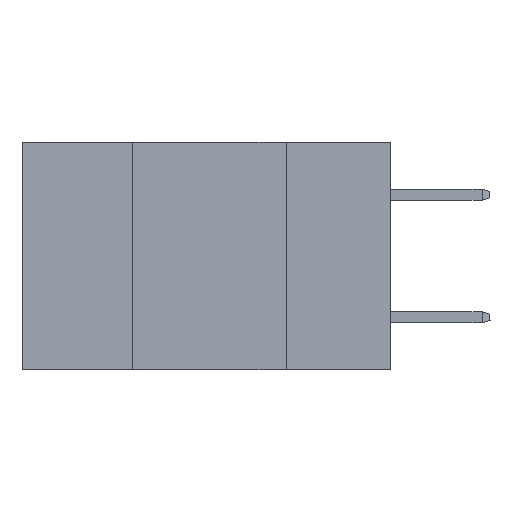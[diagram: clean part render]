
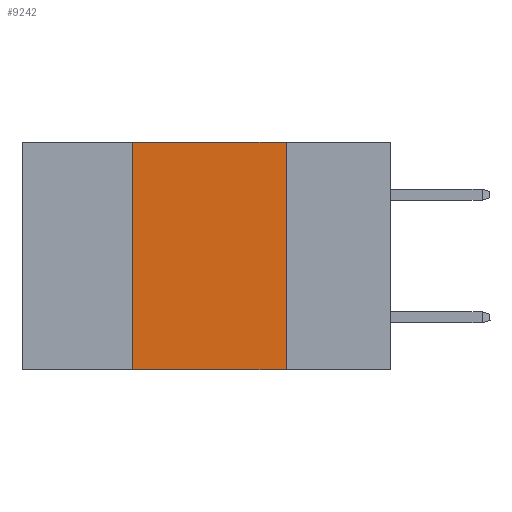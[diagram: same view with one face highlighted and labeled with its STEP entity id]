
A CAD part, left-side view. The second image highlights one B-rep face of the part: STEP entity #9242.
In plain terms, the highlighted planar face has unit normal (-1, 0, 0).
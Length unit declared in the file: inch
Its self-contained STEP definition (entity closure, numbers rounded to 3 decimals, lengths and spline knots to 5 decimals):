
#1092 = EDGE_CURVE ( 'NONE', #11056, #17982, #3952, .T. ) ;
#1175 = DIRECTION ( 'NONE',  ( 1., 0., 0. ) ) ;
#1371 = DIRECTION ( 'NONE',  ( 0., 0., -1. ) ) ;
#1800 = CARTESIAN_POINT ( 'NONE',  ( 0., 0.42, -0.37 ) ) ;
#2839 = VECTOR ( 'NONE', #8505, 39.37008 ) ;
#3799 = ORIENTED_EDGE ( 'NONE', *, *, #16198, .F. ) ;
#3952 = LINE ( 'NONE', #16289, #2839 ) ;
#5340 = EDGE_LOOP ( 'NONE', ( #8524, #3799, #18509, #17405 ) ) ;
#5628 = LINE ( 'NONE', #19074, #18028 ) ;
#5775 = CARTESIAN_POINT ( 'NONE',  ( 0., 0.17, 0. ) ) ;
#7047 = DIRECTION ( 'NONE',  ( 0., 0., 1. ) ) ;
#7302 = FACE_OUTER_BOUND ( 'NONE', #5340, .T. ) ;
#7561 = AXIS2_PLACEMENT_3D ( 'NONE', #8721, #1175, #1371 ) ;
#8074 = CARTESIAN_POINT ( 'NONE',  ( 0., 0.6, 0. ) ) ;
#8477 = VERTEX_POINT ( 'NONE', #1800 ) ;
#8505 = DIRECTION ( 'NONE',  ( 0., 0., -1. ) ) ;
#8524 = ORIENTED_EDGE ( 'NONE', *, *, #1092, .F. ) ;
#8721 = CARTESIAN_POINT ( 'NONE',  ( 0., 0.6, 0. ) ) ;
#9242 = ADVANCED_FACE ( 'NONE', ( #7302 ), #13471, .F. ) ;
#11056 = VERTEX_POINT ( 'NONE', #5775 ) ;
#11897 = LINE ( 'NONE', #18059, #19009 ) ;
#12640 = DIRECTION ( 'NONE',  ( 0., -1., 0. ) ) ;
#13471 = PLANE ( 'NONE',  #7561 ) ;
#13657 = VERTEX_POINT ( 'NONE', #16832 ) ;
#13703 = DIRECTION ( 'NONE',  ( 0., -1., 0. ) ) ;
#14774 = CARTESIAN_POINT ( 'NONE',  ( 0., 0.17, -0.37 ) ) ;
#15655 = EDGE_CURVE ( 'NONE', #8477, #17982, #11897, .T. ) ;
#15668 = LINE ( 'NONE', #8074, #17746 ) ;
#16198 = EDGE_CURVE ( 'NONE', #13657, #11056, #15668, .T. ) ;
#16289 = CARTESIAN_POINT ( 'NONE',  ( 0., 0.17, 0. ) ) ;
#16832 = CARTESIAN_POINT ( 'NONE',  ( 0., 0.42, 0. ) ) ;
#16865 = EDGE_CURVE ( 'NONE', #8477, #13657, #5628, .T. ) ;
#17405 = ORIENTED_EDGE ( 'NONE', *, *, #15655, .T. ) ;
#17746 = VECTOR ( 'NONE', #12640, 39.37008 ) ;
#17982 = VERTEX_POINT ( 'NONE', #14774 ) ;
#18028 = VECTOR ( 'NONE', #7047, 39.37008 ) ;
#18059 = CARTESIAN_POINT ( 'NONE',  ( 0., 0.6, -0.37 ) ) ;
#18509 = ORIENTED_EDGE ( 'NONE', *, *, #16865, .F. ) ;
#19009 = VECTOR ( 'NONE', #13703, 39.37008 ) ;
#19074 = CARTESIAN_POINT ( 'NONE',  ( 0., 0.42, 0. ) ) ;
